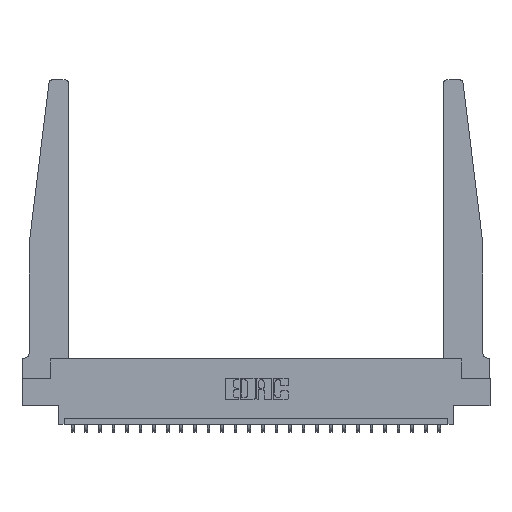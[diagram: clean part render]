
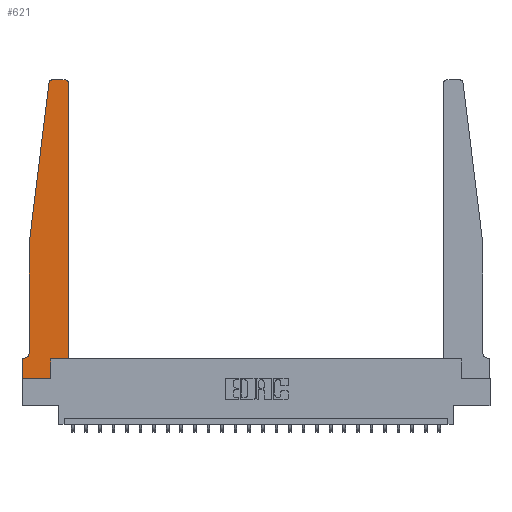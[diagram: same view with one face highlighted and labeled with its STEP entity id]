
A CAD part, top view. The second image highlights one B-rep face of the part: STEP entity #621.
In plain terms, the highlighted planar face has unit normal (0, 0, 1).
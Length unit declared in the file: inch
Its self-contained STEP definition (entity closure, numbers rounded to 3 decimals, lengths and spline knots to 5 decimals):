
#621 = ADVANCED_FACE ( 'NONE', ( #19920 ), #1064, .T. ) ;
#713 = LINE ( 'NONE', #2573, #3520 ) ;
#1047 = VERTEX_POINT ( 'NONE', #6145 ) ;
#1064 = PLANE ( 'NONE',  #8796 ) ;
#1735 = ORIENTED_EDGE ( 'NONE', *, *, #12092, .T. ) ;
#1992 = VECTOR ( 'NONE', #20622, 39.37008 ) ;
#2226 = CARTESIAN_POINT ( 'NONE',  ( 0.25, 2.75, 0.37 ) ) ;
#2261 = AXIS2_PLACEMENT_3D ( 'NONE', #15740, #23363, #13887 ) ;
#2332 = VERTEX_POINT ( 'NONE', #4767 ) ;
#2573 = CARTESIAN_POINT ( 'NONE',  ( 0.425, 0.18, 0.37 ) ) ;
#2726 = ORIENTED_EDGE ( 'NONE', *, *, #12988, .T. ) ;
#3520 = VECTOR ( 'NONE', #4935, 39.37008 ) ;
#3593 = ORIENTED_EDGE ( 'NONE', *, *, #6652, .T. ) ;
#3713 = VERTEX_POINT ( 'NONE', #23463 ) ;
#4297 = ORIENTED_EDGE ( 'NONE', *, *, #15248, .T. ) ;
#4478 = CIRCLE ( 'NONE', #6868, 0.03 ) ;
#4579 = CARTESIAN_POINT ( 'NONE',  ( 0.425, 0.18, 0.37 ) ) ;
#4670 = DIRECTION ( 'NONE',  ( 1., 0., 0. ) ) ;
#4767 = CARTESIAN_POINT ( 'NONE',  ( 0., 0.1875, 0.37 ) ) ;
#4803 = EDGE_CURVE ( 'NONE', #1047, #15619, #11529, .T. ) ;
#4921 = VERTEX_POINT ( 'NONE', #6632 ) ;
#4935 = DIRECTION ( 'NONE',  ( 1., 0., 0. ) ) ;
#5090 = ORIENTED_EDGE ( 'NONE', *, *, #18084, .T. ) ;
#5606 = DIRECTION ( 'NONE',  ( 0., 0., -1. ) ) ;
#5973 = CARTESIAN_POINT ( 'NONE',  ( 0.015, 0.2375, 0.37 ) ) ;
#6145 = CARTESIAN_POINT ( 'NONE',  ( 0.24675, 2.72367, 0.37 ) ) ;
#6632 = CARTESIAN_POINT ( 'NONE',  ( 0.015, 0.1875, 0.37 ) ) ;
#6643 = CIRCLE ( 'NONE', #20216, 0.05 ) ;
#6652 = EDGE_CURVE ( 'NONE', #12850, #1047, #4478, .T. ) ;
#6868 = AXIS2_PLACEMENT_3D ( 'NONE', #7466, #18842, #16837 ) ;
#7138 = DIRECTION ( 'NONE',  ( 0., -1., 0. ) ) ;
#7466 = CARTESIAN_POINT ( 'NONE',  ( 0.27653, 2.72, 0.37 ) ) ;
#7721 = CARTESIAN_POINT ( 'NONE',  ( 0.2605, 0., 0.37 ) ) ;
#7918 = VERTEX_POINT ( 'NONE', #20833 ) ;
#7997 = CARTESIAN_POINT ( 'NONE',  ( 0.27653, 2.75, 0.37 ) ) ;
#8121 = DIRECTION ( 'NONE',  ( 1., 0., 0. ) ) ;
#8186 = ORIENTED_EDGE ( 'NONE', *, *, #4803, .T. ) ;
#8457 = DIRECTION ( 'NONE',  ( -1., 0., 0. ) ) ;
#8537 = VECTOR ( 'NONE', #24029, 39.37008 ) ;
#8612 = VECTOR ( 'NONE', #8457, 39.37008 ) ;
#8646 = CIRCLE ( 'NONE', #2261, 0.03 ) ;
#8675 = DIRECTION ( 'NONE',  ( 0., 0., 1. ) ) ;
#8686 = ORIENTED_EDGE ( 'NONE', *, *, #13008, .T. ) ;
#8796 = AXIS2_PLACEMENT_3D ( 'NONE', #17667, #8675, #4670 ) ;
#9007 = CARTESIAN_POINT ( 'NONE',  ( 0.065, 0.1875, 0.37 ) ) ;
#9136 = CARTESIAN_POINT ( 'NONE',  ( 0.065, 1.25, 0.37 ) ) ;
#9155 = ORIENTED_EDGE ( 'NONE', *, *, #23145, .T. ) ;
#9373 = VERTEX_POINT ( 'NONE', #4579 ) ;
#9997 = LINE ( 'NONE', #17615, #17828 ) ;
#10183 = CARTESIAN_POINT ( 'NONE',  ( 0.425, 2.72, 0.37 ) ) ;
#10314 = DIRECTION ( 'NONE',  ( 0., -1., 0. ) ) ;
#10413 = VECTOR ( 'NONE', #10314, 39.37008 ) ;
#10420 = ORIENTED_EDGE ( 'NONE', *, *, #11591, .T. ) ;
#10557 = CARTESIAN_POINT ( 'NONE',  ( 0., 0., 0.37 ) ) ;
#11391 = ORIENTED_EDGE ( 'NONE', *, *, #17409, .T. ) ;
#11461 = CARTESIAN_POINT ( 'NONE',  ( 0.2605, 0.18, 0.37 ) ) ;
#11529 = LINE ( 'NONE', #11901, #18378 ) ;
#11591 = EDGE_CURVE ( 'NONE', #15619, #19800, #16634, .T. ) ;
#11901 = CARTESIAN_POINT ( 'NONE',  ( 0.065, 1.25, 0.37 ) ) ;
#12092 = EDGE_CURVE ( 'NONE', #20571, #12850, #13847, .T. ) ;
#12850 = VERTEX_POINT ( 'NONE', #7997 ) ;
#12988 = EDGE_CURVE ( 'NONE', #7918, #22339, #9997, .T. ) ;
#13008 = EDGE_CURVE ( 'NONE', #16947, #20571, #8646, .T. ) ;
#13187 = EDGE_CURVE ( 'NONE', #19800, #4921, #6643, .T. ) ;
#13335 = LINE ( 'NONE', #11461, #19049 ) ;
#13458 = DIRECTION ( 'NONE',  ( 0., 1., 0. ) ) ;
#13648 = EDGE_LOOP ( 'NONE', ( #1735, #3593, #8186, #10420, #18706, #11391, #5090, #2726, #22124, #4297, #9155, #8686 ) ) ;
#13794 = EDGE_CURVE ( 'NONE', #22339, #3713, #13335, .T. ) ;
#13847 = LINE ( 'NONE', #2226, #8612 ) ;
#13887 = DIRECTION ( 'NONE',  ( 1., 0., 0. ) ) ;
#13898 = DIRECTION ( 'NONE',  ( -0.122, -0.992, 0. ) ) ;
#15248 = EDGE_CURVE ( 'NONE', #3713, #9373, #713, .T. ) ;
#15619 = VERTEX_POINT ( 'NONE', #24670 ) ;
#15740 = CARTESIAN_POINT ( 'NONE',  ( 0.395, 2.72, 0.37 ) ) ;
#15759 = LINE ( 'NONE', #9007, #1992 ) ;
#16181 = LINE ( 'NONE', #23794, #8537 ) ;
#16634 = LINE ( 'NONE', #9136, #16968 ) ;
#16837 = DIRECTION ( 'NONE',  ( 1., 0., 0. ) ) ;
#16947 = VERTEX_POINT ( 'NONE', #10183 ) ;
#16968 = VECTOR ( 'NONE', #7138, 39.37008 ) ;
#17409 = EDGE_CURVE ( 'NONE', #4921, #2332, #15759, .T. ) ;
#17615 = CARTESIAN_POINT ( 'NONE',  ( 0., 0., 0.37 ) ) ;
#17667 = CARTESIAN_POINT ( 'NONE',  ( 0., 0.1875, 0.37 ) ) ;
#17828 = VECTOR ( 'NONE', #8121, 39.37008 ) ;
#18084 = EDGE_CURVE ( 'NONE', #2332, #7918, #23791, .T. ) ;
#18378 = VECTOR ( 'NONE', #13898, 39.37008 ) ;
#18706 = ORIENTED_EDGE ( 'NONE', *, *, #13187, .T. ) ;
#18842 = DIRECTION ( 'NONE',  ( 0., 0., 1. ) ) ;
#19049 = VECTOR ( 'NONE', #13458, 39.37008 ) ;
#19117 = CARTESIAN_POINT ( 'NONE',  ( 0.065, 0.2375, 0.37 ) ) ;
#19800 = VERTEX_POINT ( 'NONE', #19117 ) ;
#19920 = FACE_OUTER_BOUND ( 'NONE', #13648, .T. ) ;
#20216 = AXIS2_PLACEMENT_3D ( 'NONE', #5973, #5606, #22843 ) ;
#20571 = VERTEX_POINT ( 'NONE', #21267 ) ;
#20622 = DIRECTION ( 'NONE',  ( -1., 0., 0. ) ) ;
#20833 = CARTESIAN_POINT ( 'NONE',  ( 0., 0., 0.37 ) ) ;
#21267 = CARTESIAN_POINT ( 'NONE',  ( 0.395, 2.75, 0.37 ) ) ;
#22124 = ORIENTED_EDGE ( 'NONE', *, *, #13794, .T. ) ;
#22339 = VERTEX_POINT ( 'NONE', #7721 ) ;
#22843 = DIRECTION ( 'NONE',  ( -1., 0., 0. ) ) ;
#23145 = EDGE_CURVE ( 'NONE', #9373, #16947, #16181, .T. ) ;
#23363 = DIRECTION ( 'NONE',  ( 0., 0., 1. ) ) ;
#23463 = CARTESIAN_POINT ( 'NONE',  ( 0.2605, 0.18, 0.37 ) ) ;
#23791 = LINE ( 'NONE', #10557, #10413 ) ;
#23794 = CARTESIAN_POINT ( 'NONE',  ( 0.425, 0.18, 0.37 ) ) ;
#24029 = DIRECTION ( 'NONE',  ( 0., 1., 0. ) ) ;
#24670 = CARTESIAN_POINT ( 'NONE',  ( 0.065, 1.25, 0.37 ) ) ;
